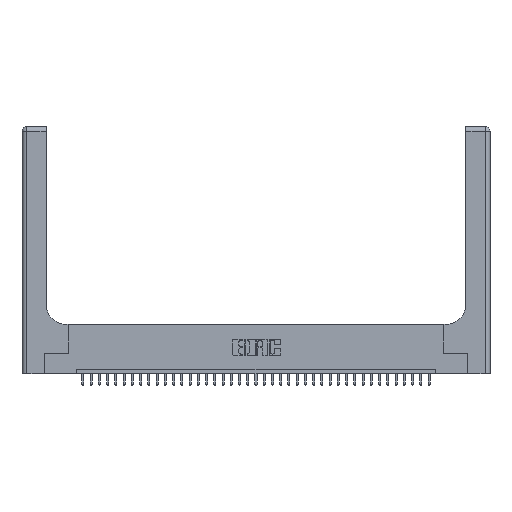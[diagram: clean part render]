
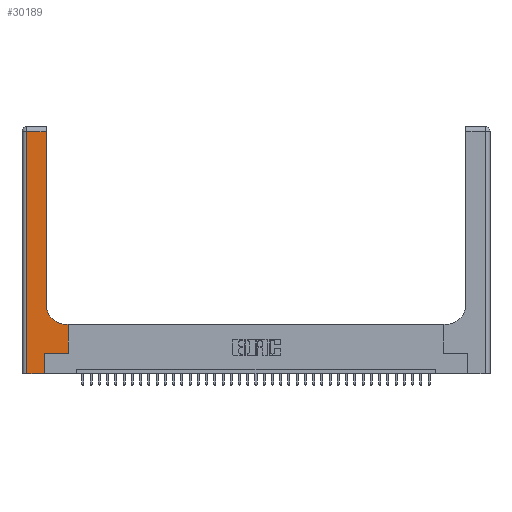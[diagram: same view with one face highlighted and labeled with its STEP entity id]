
A CAD part, top view. The second image highlights one B-rep face of the part: STEP entity #30189.
In plain terms, the highlighted planar face has unit normal (0, 0, 1).
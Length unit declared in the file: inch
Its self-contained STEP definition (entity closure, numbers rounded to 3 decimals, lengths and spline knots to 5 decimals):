
#471 = VECTOR ( 'NONE', #36164, 39.37008 ) ;
#1419 = LINE ( 'NONE', #7210, #471 ) ;
#2110 = DIRECTION ( 'NONE',  ( 0., 1., 0. ) ) ;
#2145 = CARTESIAN_POINT ( 'NONE',  ( 0.2915, 2.94, 0.37 ) ) ;
#2336 = EDGE_CURVE ( 'NONE', #13890, #8665, #1419, .T. ) ;
#2474 = CARTESIAN_POINT ( 'NONE',  ( 0.5415, 0.6, 0.37 ) ) ;
#2978 = CARTESIAN_POINT ( 'NONE',  ( 0.2915, 0.85, 0.37 ) ) ;
#3511 = DIRECTION ( 'NONE',  ( -1., 0., 0. ) ) ;
#3838 = VECTOR ( 'NONE', #9642, 39.37008 ) ;
#4089 = VECTOR ( 'NONE', #26751, 39.37008 ) ;
#4247 = CARTESIAN_POINT ( 'NONE',  ( 0., 3., 0.37 ) ) ;
#4265 = DIRECTION ( 'NONE',  ( 0., 0., -1. ) ) ;
#4759 = AXIS2_PLACEMENT_3D ( 'NONE', #4247, #26862, #15636 ) ;
#4819 = EDGE_CURVE ( 'NONE', #18434, #13890, #20279, .T. ) ;
#5304 = LINE ( 'NONE', #10682, #30587 ) ;
#7015 = LINE ( 'NONE', #20499, #35961 ) ;
#7210 = CARTESIAN_POINT ( 'NONE',  ( 0.2915, 3., 0.37 ) ) ;
#7277 = EDGE_LOOP ( 'NONE', ( #32524, #35015, #30877, #28887, #22060, #14156, #25994, #22158, #32283 ) ) ;
#7724 = EDGE_CURVE ( 'NONE', #8627, #30417, #12443, .T. ) ;
#7791 = DIRECTION ( 'NONE',  ( 1., 0., 0. ) ) ;
#8173 = CARTESIAN_POINT ( 'NONE',  ( 0.269, 0., 0.37 ) ) ;
#8627 = VERTEX_POINT ( 'NONE', #17094 ) ;
#8665 = VERTEX_POINT ( 'NONE', #2145 ) ;
#9190 = CARTESIAN_POINT ( 'NONE',  ( 0., 2.94, 0.37 ) ) ;
#9515 = VECTOR ( 'NONE', #3511, 39.37008 ) ;
#9642 = DIRECTION ( 'NONE',  ( 1., 0., 0. ) ) ;
#9750 = CARTESIAN_POINT ( 'NONE',  ( 0.5585, 0.25, 0.37 ) ) ;
#10457 = LINE ( 'NONE', #15399, #9515 ) ;
#10682 = CARTESIAN_POINT ( 'NONE',  ( 0.5585, 0.25, 0.37 ) ) ;
#11077 = EDGE_CURVE ( 'NONE', #28933, #18434, #10457, .T. ) ;
#11778 = DIRECTION ( 'NONE',  ( 0., 1., 0. ) ) ;
#12283 = CARTESIAN_POINT ( 'NONE',  ( 0., 0., 0.37 ) ) ;
#12443 = LINE ( 'NONE', #12283, #3838 ) ;
#12937 = EDGE_CURVE ( 'NONE', #30417, #19210, #7015, .T. ) ;
#13890 = VERTEX_POINT ( 'NONE', #2978 ) ;
#14156 = ORIENTED_EDGE ( 'NONE', *, *, #37226, .T. ) ;
#14687 = AXIS2_PLACEMENT_3D ( 'NONE', #33035, #4265, #24501 ) ;
#15399 = CARTESIAN_POINT ( 'NONE',  ( 0.2915, 0.6, 0.37 ) ) ;
#15636 = DIRECTION ( 'NONE',  ( -1., 0., 0. ) ) ;
#17094 = CARTESIAN_POINT ( 'NONE',  ( 0.06, 0., 0.37 ) ) ;
#18434 = VERTEX_POINT ( 'NONE', #2474 ) ;
#19210 = VERTEX_POINT ( 'NONE', #33054 ) ;
#19787 = EDGE_CURVE ( 'NONE', #25985, #8627, #30340, .T. ) ;
#20267 = EDGE_CURVE ( 'NONE', #8665, #25985, #22225, .T. ) ;
#20279 = CIRCLE ( 'NONE', #14687, 0.25 ) ;
#20499 = CARTESIAN_POINT ( 'NONE',  ( 0.269, 0., 0.37 ) ) ;
#22060 = ORIENTED_EDGE ( 'NONE', *, *, #12937, .T. ) ;
#22158 = ORIENTED_EDGE ( 'NONE', *, *, #11077, .T. ) ;
#22225 = LINE ( 'NONE', #9190, #4089 ) ;
#23279 = LINE ( 'NONE', #27871, #25581 ) ;
#24065 = CARTESIAN_POINT ( 'NONE',  ( 0.5585, 0.6, 0.37 ) ) ;
#24501 = DIRECTION ( 'NONE',  ( 1., 0., 0. ) ) ;
#25581 = VECTOR ( 'NONE', #7791, 39.37008 ) ;
#25985 = VERTEX_POINT ( 'NONE', #31501 ) ;
#25994 = ORIENTED_EDGE ( 'NONE', *, *, #30785, .T. ) ;
#26295 = VECTOR ( 'NONE', #30153, 39.37008 ) ;
#26751 = DIRECTION ( 'NONE',  ( -1., 0., 0. ) ) ;
#26862 = DIRECTION ( 'NONE',  ( 0., 0., -1. ) ) ;
#27871 = CARTESIAN_POINT ( 'NONE',  ( 0.269, 0.25, 0.37 ) ) ;
#28887 = ORIENTED_EDGE ( 'NONE', *, *, #7724, .T. ) ;
#28933 = VERTEX_POINT ( 'NONE', #24065 ) ;
#30153 = DIRECTION ( 'NONE',  ( 0., -1., 0. ) ) ;
#30189 = ADVANCED_FACE ( 'NONE', ( #34675 ), #32760, .F. ) ;
#30340 = LINE ( 'NONE', #31456, #26295 ) ;
#30417 = VERTEX_POINT ( 'NONE', #8173 ) ;
#30587 = VECTOR ( 'NONE', #2110, 39.37008 ) ;
#30785 = EDGE_CURVE ( 'NONE', #31556, #28933, #5304, .T. ) ;
#30877 = ORIENTED_EDGE ( 'NONE', *, *, #19787, .T. ) ;
#31456 = CARTESIAN_POINT ( 'NONE',  ( 0.06, 3., 0.37 ) ) ;
#31501 = CARTESIAN_POINT ( 'NONE',  ( 0.06, 2.94, 0.37 ) ) ;
#31556 = VERTEX_POINT ( 'NONE', #9750 ) ;
#32283 = ORIENTED_EDGE ( 'NONE', *, *, #4819, .T. ) ;
#32524 = ORIENTED_EDGE ( 'NONE', *, *, #2336, .T. ) ;
#32760 = PLANE ( 'NONE',  #4759 ) ;
#33035 = CARTESIAN_POINT ( 'NONE',  ( 0.5415, 0.85, 0.37 ) ) ;
#33054 = CARTESIAN_POINT ( 'NONE',  ( 0.269, 0.25, 0.37 ) ) ;
#34675 = FACE_OUTER_BOUND ( 'NONE', #7277, .T. ) ;
#35015 = ORIENTED_EDGE ( 'NONE', *, *, #20267, .T. ) ;
#35961 = VECTOR ( 'NONE', #11778, 39.37008 ) ;
#36164 = DIRECTION ( 'NONE',  ( 0., 1., 0. ) ) ;
#37226 = EDGE_CURVE ( 'NONE', #19210, #31556, #23279, .T. ) ;
